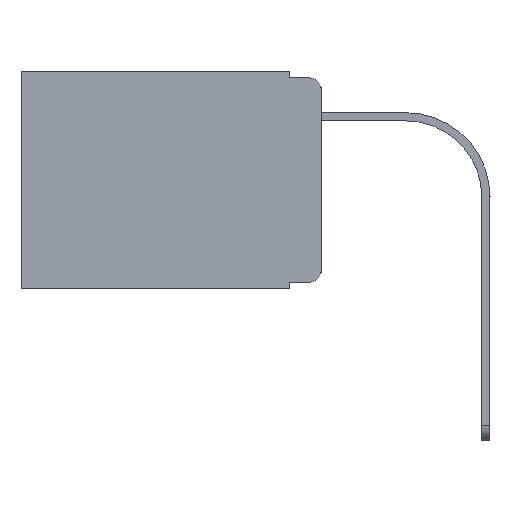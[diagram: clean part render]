
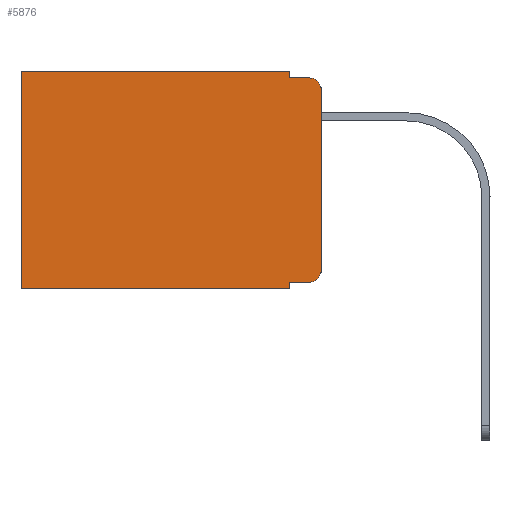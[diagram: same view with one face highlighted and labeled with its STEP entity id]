
A CAD part, left-side view. The second image highlights one B-rep face of the part: STEP entity #5876.
In plain terms, the highlighted planar face has unit normal (-1, 0, 0).
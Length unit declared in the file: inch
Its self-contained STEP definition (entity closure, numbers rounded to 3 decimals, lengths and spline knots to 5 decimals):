
#53 = EDGE_LOOP ( 'NONE', ( #5322, #8178, #3949, #1303, #1053, #9394, #5523, #244, #7593, #6727 ) ) ;
#84 = VECTOR ( 'NONE', #7339, 39.37008 ) ;
#126 = CARTESIAN_POINT ( 'NONE',  ( 0.298, 0.051, 0. ) ) ;
#244 = ORIENTED_EDGE ( 'NONE', *, *, #3231, .F. ) ;
#741 = LINE ( 'NONE', #7452, #4988 ) ;
#795 = DIRECTION ( 'NONE',  ( 0., 1., 0. ) ) ;
#810 = VERTEX_POINT ( 'NONE', #4279 ) ;
#972 = LINE ( 'NONE', #3895, #5206 ) ;
#1053 = ORIENTED_EDGE ( 'NONE', *, *, #5344, .T. ) ;
#1160 = FACE_OUTER_BOUND ( 'NONE', #53, .T. ) ;
#1207 = EDGE_CURVE ( 'NONE', #1772, #8170, #3841, .T. ) ;
#1219 = EDGE_CURVE ( 'NONE', #4374, #3819, #9342, .T. ) ;
#1303 = ORIENTED_EDGE ( 'NONE', *, *, #4242, .F. ) ;
#1340 = CARTESIAN_POINT ( 'NONE',  ( 0.298, 0.051, -0.01 ) ) ;
#1348 = LINE ( 'NONE', #4380, #2312 ) ;
#1426 = VECTOR ( 'NONE', #6339, 39.37008 ) ;
#1772 = VERTEX_POINT ( 'NONE', #3035 ) ;
#1829 = CARTESIAN_POINT ( 'NONE',  ( 0.298, 0., -0.313 ) ) ;
#1830 = DIRECTION ( 'NONE',  ( 1., 0., 0. ) ) ;
#2206 = VECTOR ( 'NONE', #6147, 39.37008 ) ;
#2220 = LINE ( 'NONE', #126, #84 ) ;
#2312 = VECTOR ( 'NONE', #5224, 39.37008 ) ;
#2674 = CARTESIAN_POINT ( 'NONE',  ( 0.298, 0.02, -0.03 ) ) ;
#2733 = EDGE_CURVE ( 'NONE', #3926, #810, #6875, .T. ) ;
#2788 = CARTESIAN_POINT ( 'NONE',  ( 0.298, 0.02, -0.313 ) ) ;
#2918 = CARTESIAN_POINT ( 'NONE',  ( 0.298, 0.02, -0.333 ) ) ;
#3035 = CARTESIAN_POINT ( 'NONE',  ( 0.298, 0., -0.03 ) ) ;
#3216 = EDGE_CURVE ( 'NONE', #7269, #810, #6101, .T. ) ;
#3231 = EDGE_CURVE ( 'NONE', #4374, #7269, #7809, .T. ) ;
#3243 = DIRECTION ( 'NONE',  ( 0., 0., -1. ) ) ;
#3265 = EDGE_CURVE ( 'NONE', #3819, #4712, #8621, .T. ) ;
#3505 = DIRECTION ( 'NONE',  ( -1., 0., 0. ) ) ;
#3677 = AXIS2_PLACEMENT_3D ( 'NONE', #4078, #1830, #8305 ) ;
#3819 = VERTEX_POINT ( 'NONE', #2918 ) ;
#3841 = CIRCLE ( 'NONE', #8575, 0.02 ) ;
#3895 = CARTESIAN_POINT ( 'NONE',  ( 0.298, 0., 0. ) ) ;
#3919 = CARTESIAN_POINT ( 'NONE',  ( 0.298, 0.02, -0.01 ) ) ;
#3926 = VERTEX_POINT ( 'NONE', #6460 ) ;
#3949 = ORIENTED_EDGE ( 'NONE', *, *, #8758, .F. ) ;
#4078 = CARTESIAN_POINT ( 'NONE',  ( 0.298, 0., 0. ) ) ;
#4212 = CARTESIAN_POINT ( 'NONE',  ( 0.298, 0.051, 0. ) ) ;
#4215 = VERTEX_POINT ( 'NONE', #1340 ) ;
#4242 = EDGE_CURVE ( 'NONE', #8809, #4215, #2220, .T. ) ;
#4279 = CARTESIAN_POINT ( 'NONE',  ( 0.298, 0.473, -0.343 ) ) ;
#4374 = VERTEX_POINT ( 'NONE', #6912 ) ;
#4380 = CARTESIAN_POINT ( 'NONE',  ( 0.298, 0.051, -0.01 ) ) ;
#4712 = VERTEX_POINT ( 'NONE', #1829 ) ;
#4988 = VECTOR ( 'NONE', #795, 39.37008 ) ;
#5206 = VECTOR ( 'NONE', #9244, 39.37008 ) ;
#5224 = DIRECTION ( 'NONE',  ( 0., -1., 0. ) ) ;
#5322 = ORIENTED_EDGE ( 'NONE', *, *, #5965, .F. ) ;
#5344 = EDGE_CURVE ( 'NONE', #8809, #3926, #741, .T. ) ;
#5499 = PLANE ( 'NONE',  #3677 ) ;
#5523 = ORIENTED_EDGE ( 'NONE', *, *, #3216, .F. ) ;
#5602 = CARTESIAN_POINT ( 'NONE',  ( 0.298, 0.051, -0.333 ) ) ;
#5710 = DIRECTION ( 'NONE',  ( 0., 0., -1. ) ) ;
#5876 = ADVANCED_FACE ( 'NONE', ( #1160 ), #5499, .F. ) ;
#5965 = EDGE_CURVE ( 'NONE', #1772, #4712, #972, .T. ) ;
#6101 = LINE ( 'NONE', #8989, #2206 ) ;
#6147 = DIRECTION ( 'NONE',  ( 0., 1., 0. ) ) ;
#6314 = DIRECTION ( 'NONE',  ( 0., -1., 0. ) ) ;
#6339 = DIRECTION ( 'NONE',  ( 0., 0., -1. ) ) ;
#6460 = CARTESIAN_POINT ( 'NONE',  ( 0.298, 0.473, 0. ) ) ;
#6727 = ORIENTED_EDGE ( 'NONE', *, *, #3265, .T. ) ;
#6875 = LINE ( 'NONE', #9145, #8456 ) ;
#6912 = CARTESIAN_POINT ( 'NONE',  ( 0.298, 0.051, -0.333 ) ) ;
#7269 = VERTEX_POINT ( 'NONE', #7412 ) ;
#7339 = DIRECTION ( 'NONE',  ( 0., 0., -1. ) ) ;
#7412 = CARTESIAN_POINT ( 'NONE',  ( 0.298, 0.051, -0.343 ) ) ;
#7452 = CARTESIAN_POINT ( 'NONE',  ( 0.298, 0., 0. ) ) ;
#7593 = ORIENTED_EDGE ( 'NONE', *, *, #1219, .T. ) ;
#7786 = DIRECTION ( 'NONE',  ( -1., 0., 0. ) ) ;
#7809 = LINE ( 'NONE', #4212, #1426 ) ;
#8170 = VERTEX_POINT ( 'NONE', #3919 ) ;
#8178 = ORIENTED_EDGE ( 'NONE', *, *, #1207, .T. ) ;
#8305 = DIRECTION ( 'NONE',  ( 0., 0., -1. ) ) ;
#8426 = VECTOR ( 'NONE', #6314, 39.37008 ) ;
#8456 = VECTOR ( 'NONE', #3243, 39.37008 ) ;
#8575 = AXIS2_PLACEMENT_3D ( 'NONE', #2674, #7786, #9383 ) ;
#8621 = CIRCLE ( 'NONE', #8625, 0.02 ) ;
#8625 = AXIS2_PLACEMENT_3D ( 'NONE', #2788, #3505, #5710 ) ;
#8758 = EDGE_CURVE ( 'NONE', #4215, #8170, #1348, .T. ) ;
#8809 = VERTEX_POINT ( 'NONE', #8825 ) ;
#8825 = CARTESIAN_POINT ( 'NONE',  ( 0.298, 0.051, 0. ) ) ;
#8989 = CARTESIAN_POINT ( 'NONE',  ( 0.298, 0., -0.343 ) ) ;
#9145 = CARTESIAN_POINT ( 'NONE',  ( 0.298, 0.473, 0. ) ) ;
#9244 = DIRECTION ( 'NONE',  ( 0., 0., -1. ) ) ;
#9342 = LINE ( 'NONE', #5602, #8426 ) ;
#9383 = DIRECTION ( 'NONE',  ( 0., 0., -1. ) ) ;
#9394 = ORIENTED_EDGE ( 'NONE', *, *, #2733, .T. ) ;
